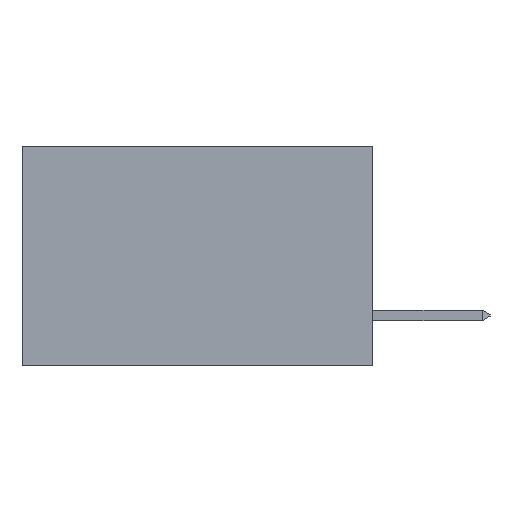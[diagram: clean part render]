
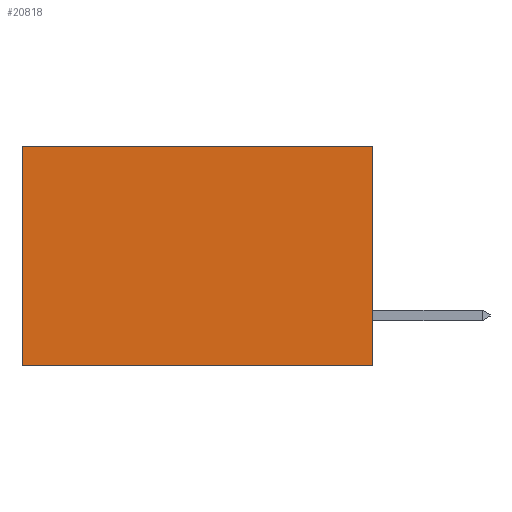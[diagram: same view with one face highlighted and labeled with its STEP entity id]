
A CAD part, left-side view. The second image highlights one B-rep face of the part: STEP entity #20818.
In plain terms, the highlighted planar face has unit normal (-1, 0, 0).
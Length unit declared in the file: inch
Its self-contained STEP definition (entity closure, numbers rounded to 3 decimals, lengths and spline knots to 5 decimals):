
#506 = AXIS2_PLACEMENT_3D ( 'NONE', #17037, #18673, #8905 ) ;
#886 = CARTESIAN_POINT ( 'NONE',  ( 0.277, 0., -0.37 ) ) ;
#1591 = LINE ( 'NONE', #2812, #14424 ) ;
#2812 = CARTESIAN_POINT ( 'NONE',  ( 0.277, 0., -0.37 ) ) ;
#2900 = VECTOR ( 'NONE', #17752, 39.37008 ) ;
#3637 = EDGE_CURVE ( 'NONE', #20386, #4812, #1591, .T. ) ;
#4324 = VECTOR ( 'NONE', #8336, 39.37008 ) ;
#4812 = VERTEX_POINT ( 'NONE', #12552 ) ;
#6037 = ORIENTED_EDGE ( 'NONE', *, *, #9958, .T. ) ;
#6245 = DIRECTION ( 'NONE',  ( 0., 1., 0. ) ) ;
#7365 = ORIENTED_EDGE ( 'NONE', *, *, #19098, .F. ) ;
#8336 = DIRECTION ( 'NONE',  ( 0., 0., -1. ) ) ;
#8416 = DIRECTION ( 'NONE',  ( 0., 1., 0. ) ) ;
#8630 = CARTESIAN_POINT ( 'NONE',  ( 0.277, 0., 0. ) ) ;
#8636 = ORIENTED_EDGE ( 'NONE', *, *, #16001, .T. ) ;
#8905 = DIRECTION ( 'NONE',  ( 0., 0., -1. ) ) ;
#9049 = VECTOR ( 'NONE', #8416, 39.37008 ) ;
#9958 = EDGE_CURVE ( 'NONE', #21276, #19981, #13445, .T. ) ;
#11090 = EDGE_LOOP ( 'NONE', ( #8636, #18620, #7365, #6037 ) ) ;
#11303 = FACE_OUTER_BOUND ( 'NONE', #11090, .T. ) ;
#11803 = CARTESIAN_POINT ( 'NONE',  ( 0.277, 0.59, 0. ) ) ;
#12552 = CARTESIAN_POINT ( 'NONE',  ( 0.277, 0.59, -0.37 ) ) ;
#13445 = LINE ( 'NONE', #8630, #9049 ) ;
#14424 = VECTOR ( 'NONE', #6245, 39.37008 ) ;
#15411 = PLANE ( 'NONE',  #506 ) ;
#16001 = EDGE_CURVE ( 'NONE', #19981, #4812, #17528, .T. ) ;
#16107 = CARTESIAN_POINT ( 'NONE',  ( 0.277, 0., -0.37 ) ) ;
#16664 = LINE ( 'NONE', #16107, #2900 ) ;
#17037 = CARTESIAN_POINT ( 'NONE',  ( 0.277, 0., -0.37 ) ) ;
#17528 = LINE ( 'NONE', #21449, #4324 ) ;
#17752 = DIRECTION ( 'NONE',  ( 0., 0., -1. ) ) ;
#18620 = ORIENTED_EDGE ( 'NONE', *, *, #3637, .F. ) ;
#18673 = DIRECTION ( 'NONE',  ( 1., 0., 0. ) ) ;
#19098 = EDGE_CURVE ( 'NONE', #21276, #20386, #16664, .T. ) ;
#19767 = CARTESIAN_POINT ( 'NONE',  ( 0.277, 0., 0. ) ) ;
#19981 = VERTEX_POINT ( 'NONE', #11803 ) ;
#20386 = VERTEX_POINT ( 'NONE', #886 ) ;
#20818 = ADVANCED_FACE ( 'NONE', ( #11303 ), #15411, .F. ) ;
#21276 = VERTEX_POINT ( 'NONE', #19767 ) ;
#21449 = CARTESIAN_POINT ( 'NONE',  ( 0.277, 0.59, -0.37 ) ) ;
